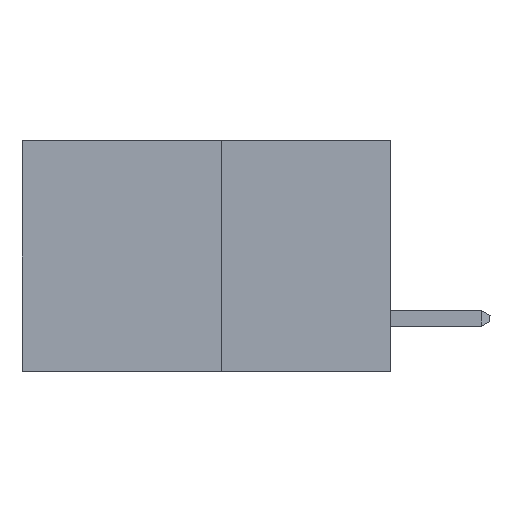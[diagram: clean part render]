
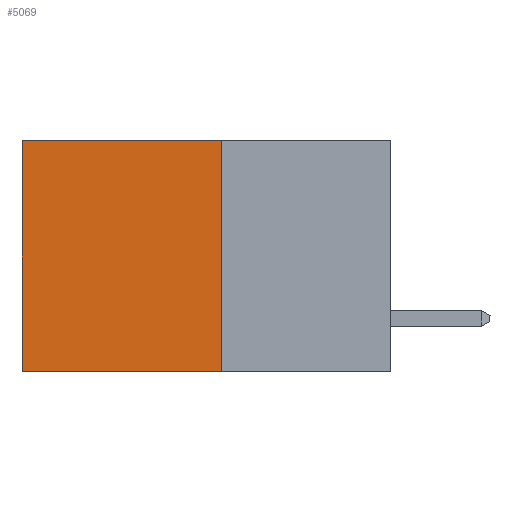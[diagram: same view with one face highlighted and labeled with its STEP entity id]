
A CAD part, left-side view. The second image highlights one B-rep face of the part: STEP entity #5069.
In plain terms, the highlighted planar face has unit normal (-1, 0, 0).
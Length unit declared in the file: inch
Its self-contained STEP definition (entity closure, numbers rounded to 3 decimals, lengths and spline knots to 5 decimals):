
#297 = CARTESIAN_POINT ( 'NONE',  ( 0.277, 0.59, -0.37 ) ) ;
#1519 = CARTESIAN_POINT ( 'NONE',  ( 0.277, 0.59, 0. ) ) ;
#1568 = DIRECTION ( 'NONE',  ( 0., 0., -1. ) ) ;
#1807 = CARTESIAN_POINT ( 'NONE',  ( 0.277, 0.59, -0.37 ) ) ;
#2357 = PLANE ( 'NONE',  #11661 ) ;
#2463 = EDGE_LOOP ( 'NONE', ( #8971, #3318, #9669, #13928 ) ) ;
#2539 = FACE_OUTER_BOUND ( 'NONE', #2463, .T. ) ;
#3274 = DIRECTION ( 'NONE',  ( 0., 1., 0. ) ) ;
#3318 = ORIENTED_EDGE ( 'NONE', *, *, #8241, .F. ) ;
#3946 = EDGE_CURVE ( 'NONE', #10658, #8589, #14550, .T. ) ;
#4673 = DIRECTION ( 'NONE',  ( 0., 0., -1. ) ) ;
#5069 = ADVANCED_FACE ( 'NONE', ( #2539 ), #2357, .F. ) ;
#5347 = EDGE_CURVE ( 'NONE', #10658, #11595, #9936, .T. ) ;
#5757 = CARTESIAN_POINT ( 'NONE',  ( 0.277, 0.27, 0. ) ) ;
#6218 = CARTESIAN_POINT ( 'NONE',  ( 0.277, 0.27, 0. ) ) ;
#6950 = VECTOR ( 'NONE', #9629, 39.37008 ) ;
#7146 = VECTOR ( 'NONE', #8391, 39.37008 ) ;
#8241 = EDGE_CURVE ( 'NONE', #8589, #14115, #14110, .T. ) ;
#8367 = CARTESIAN_POINT ( 'NONE',  ( 0.277, 0.27, -0.37 ) ) ;
#8391 = DIRECTION ( 'NONE',  ( 0., 0., -1. ) ) ;
#8412 = CARTESIAN_POINT ( 'NONE',  ( 0.277, 0.27, -0.37 ) ) ;
#8589 = VERTEX_POINT ( 'NONE', #8367 ) ;
#8971 = ORIENTED_EDGE ( 'NONE', *, *, #10838, .T. ) ;
#9484 = VECTOR ( 'NONE', #1568, 39.37008 ) ;
#9629 = DIRECTION ( 'NONE',  ( 0., 1., 0. ) ) ;
#9669 = ORIENTED_EDGE ( 'NONE', *, *, #3946, .F. ) ;
#9782 = LINE ( 'NONE', #297, #7146 ) ;
#9936 = LINE ( 'NONE', #6218, #6950 ) ;
#10230 = CARTESIAN_POINT ( 'NONE',  ( 0.277, 0.27, -0.37 ) ) ;
#10658 = VERTEX_POINT ( 'NONE', #5757 ) ;
#10838 = EDGE_CURVE ( 'NONE', #11595, #14115, #9782, .T. ) ;
#10875 = VECTOR ( 'NONE', #3274, 39.37008 ) ;
#11033 = CARTESIAN_POINT ( 'NONE',  ( 0.277, 0.27, -0.37 ) ) ;
#11313 = DIRECTION ( 'NONE',  ( 1., 0., 0. ) ) ;
#11595 = VERTEX_POINT ( 'NONE', #1519 ) ;
#11661 = AXIS2_PLACEMENT_3D ( 'NONE', #10230, #11313, #4673 ) ;
#13928 = ORIENTED_EDGE ( 'NONE', *, *, #5347, .T. ) ;
#14110 = LINE ( 'NONE', #11033, #10875 ) ;
#14115 = VERTEX_POINT ( 'NONE', #1807 ) ;
#14550 = LINE ( 'NONE', #8412, #9484 ) ;
